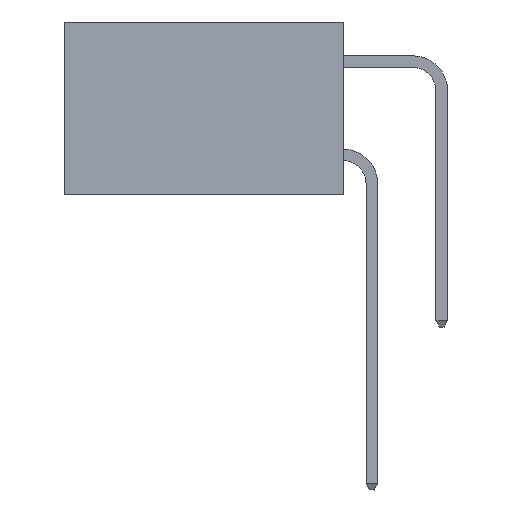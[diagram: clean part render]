
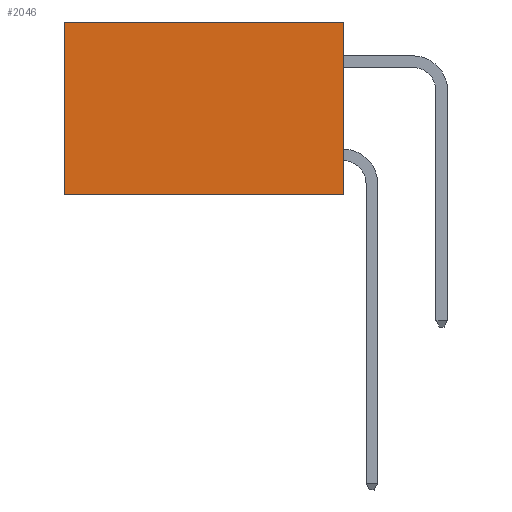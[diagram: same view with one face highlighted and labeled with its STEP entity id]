
A CAD part, left-side view. The second image highlights one B-rep face of the part: STEP entity #2046.
In plain terms, the highlighted planar face has unit normal (-1, 0, 0).
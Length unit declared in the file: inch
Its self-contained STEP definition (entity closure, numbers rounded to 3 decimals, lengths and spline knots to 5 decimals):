
#37 = CARTESIAN_POINT ( 'NONE',  ( 0.2615, 0., 0. ) ) ;
#191 = EDGE_LOOP ( 'NONE', ( #6160, #8755, #4606, #4173 ) ) ;
#199 = DIRECTION ( 'NONE',  ( 0., 0., -1. ) ) ;
#441 = FACE_OUTER_BOUND ( 'NONE', #191, .T. ) ;
#1089 = EDGE_CURVE ( 'NONE', #4806, #9891, #9917, .T. ) ;
#1210 = VECTOR ( 'NONE', #2527, 39.37008 ) ;
#1398 = CARTESIAN_POINT ( 'NONE',  ( 0.2615, 0., -0.37 ) ) ;
#1765 = CARTESIAN_POINT ( 'NONE',  ( 0.2615, 0.6, -0.37 ) ) ;
#1928 = CARTESIAN_POINT ( 'NONE',  ( 0.2615, 0.6, 0. ) ) ;
#2046 = ADVANCED_FACE ( 'NONE', ( #441 ), #7094, .F. ) ;
#2242 = VECTOR ( 'NONE', #7710, 39.37008 ) ;
#2521 = DIRECTION ( 'NONE',  ( 1., 0., 0. ) ) ;
#2527 = DIRECTION ( 'NONE',  ( 0., 0., -1. ) ) ;
#2879 = LINE ( 'NONE', #1398, #2242 ) ;
#2927 = CARTESIAN_POINT ( 'NONE',  ( 0.2615, 0., 0. ) ) ;
#3017 = EDGE_CURVE ( 'NONE', #4806, #5755, #8114, .T. ) ;
#3260 = VECTOR ( 'NONE', #6181, 39.37008 ) ;
#4173 = ORIENTED_EDGE ( 'NONE', *, *, #1089, .T. ) ;
#4279 = EDGE_CURVE ( 'NONE', #5755, #8584, #2879, .T. ) ;
#4606 = ORIENTED_EDGE ( 'NONE', *, *, #3017, .F. ) ;
#4806 = VERTEX_POINT ( 'NONE', #2927 ) ;
#4904 = DIRECTION ( 'NONE',  ( 0., 1., 0. ) ) ;
#5287 = CARTESIAN_POINT ( 'NONE',  ( 0.2615, 0., -0.37 ) ) ;
#5755 = VERTEX_POINT ( 'NONE', #5287 ) ;
#6160 = ORIENTED_EDGE ( 'NONE', *, *, #8831, .T. ) ;
#6181 = DIRECTION ( 'NONE',  ( 0., 0., -1. ) ) ;
#7094 = PLANE ( 'NONE',  #8514 ) ;
#7181 = VECTOR ( 'NONE', #4904, 39.37008 ) ;
#7710 = DIRECTION ( 'NONE',  ( 0., 1., 0. ) ) ;
#8114 = LINE ( 'NONE', #9508, #1210 ) ;
#8514 = AXIS2_PLACEMENT_3D ( 'NONE', #8633, #2521, #199 ) ;
#8536 = LINE ( 'NONE', #9924, #3260 ) ;
#8584 = VERTEX_POINT ( 'NONE', #1765 ) ;
#8633 = CARTESIAN_POINT ( 'NONE',  ( 0.2615, 0., -0.37 ) ) ;
#8755 = ORIENTED_EDGE ( 'NONE', *, *, #4279, .F. ) ;
#8831 = EDGE_CURVE ( 'NONE', #9891, #8584, #8536, .T. ) ;
#9508 = CARTESIAN_POINT ( 'NONE',  ( 0.2615, 0., -0.37 ) ) ;
#9891 = VERTEX_POINT ( 'NONE', #1928 ) ;
#9917 = LINE ( 'NONE', #37, #7181 ) ;
#9924 = CARTESIAN_POINT ( 'NONE',  ( 0.2615, 0.6, -0.37 ) ) ;
